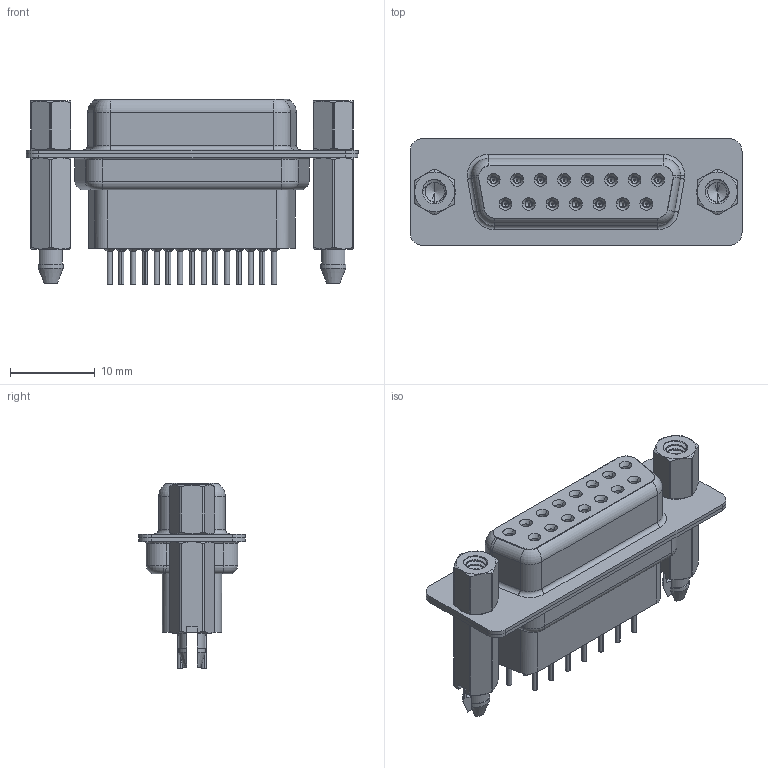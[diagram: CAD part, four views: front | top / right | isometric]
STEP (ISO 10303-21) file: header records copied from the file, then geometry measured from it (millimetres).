
FILE_DESCRIPTION (( 'STEP AP203' ), '1' );
FILE_NAME ('628-015-221-257.STEP', '2020-07-13T23:41:11', ( '' ), ( '' ), 'SwSTEP 2.0', 'SolidWorks 2020', '' );
FILE_SCHEMA (( 'CONFIG_CONTROL_DESIGN' ));
Length unit declared in the file: millimetre
Products named in the file (8): 628 Shell Front_15 Contacts; 628 Housing_15 HP; 628 4-40 Hex Standoff; 628 Contact Row 2_21H; 628 4-40 Threaded Boardlock_HP; 628-015-221-257; 628 Shell Rear_15 Contacts; 628 Contact Row 1_21H
Assembly tree (22 placements, depth 2):
  628-015-221-257
    628 Housing_15 HP
    628 Shell Front_15 Contacts
    628 Shell Rear_15 Contacts
    628 Contact Row 1_21H  x8
    628 Contact Row 2_21H  x7
    628 4-40 Hex Standoff  x2
    628 4-40 Threaded Boardlock_HP  x2
Bounding box: 39.15 x 12.6 x 21.9 mm (x, y, z)
Volume: 3736 mm3; surface area: 8710.1 mm2
Topology: 22 solids, 22 shells, 2364 faces, 6125 edges, 3844 vertices
Faces by surface type: cylinder 772, plane 586, torus 423, bspline 322, cone 261
Entity records: 32304 total; most frequent: CARTESIAN_POINT 12813, ORIENTED_EDGE 3892, DIRECTION 3819, EDGE_CURVE 1946, AXIS2_PLACEMENT_3D 1566, VERTEX_POINT 1234, EDGE_LOOP 880, CIRCLE 811
